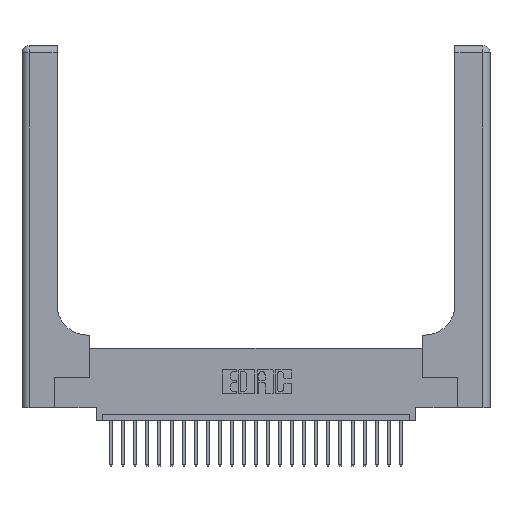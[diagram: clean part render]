
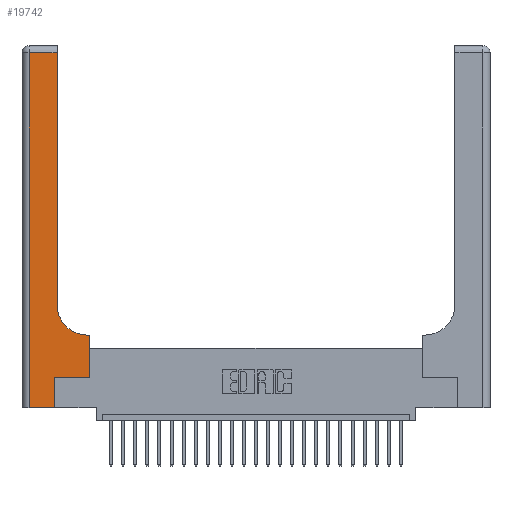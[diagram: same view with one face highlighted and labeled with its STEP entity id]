
A CAD part, top view. The second image highlights one B-rep face of the part: STEP entity #19742.
In plain terms, the highlighted planar face has unit normal (0, 0, 1).
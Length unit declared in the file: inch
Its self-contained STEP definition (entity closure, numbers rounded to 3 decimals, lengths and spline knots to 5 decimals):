
#167 = DIRECTION ( 'NONE',  ( -1., 0., 0. ) ) ;
#295 = AXIS2_PLACEMENT_3D ( 'NONE', #11099, #20944, #6883 ) ;
#512 = DIRECTION ( 'NONE',  ( 0., 1., 0. ) ) ;
#840 = DIRECTION ( 'NONE',  ( 0., 1., 0. ) ) ;
#987 = ORIENTED_EDGE ( 'NONE', *, *, #4149, .T. ) ;
#1193 = EDGE_CURVE ( 'NONE', #26446, #3257, #25566, .T. ) ;
#1522 = CARTESIAN_POINT ( 'NONE',  ( 0.269, 0.25, 0.37 ) ) ;
#2571 = LINE ( 'NONE', #17048, #23633 ) ;
#2656 = LINE ( 'NONE', #3651, #12522 ) ;
#3183 = EDGE_CURVE ( 'NONE', #15405, #6503, #21629, .T. ) ;
#3257 = VERTEX_POINT ( 'NONE', #11018 ) ;
#3651 = CARTESIAN_POINT ( 'NONE',  ( 0., 0., 0.37 ) ) ;
#4149 = EDGE_CURVE ( 'NONE', #6503, #6790, #21908, .T. ) ;
#5219 = ORIENTED_EDGE ( 'NONE', *, *, #18843, .T. ) ;
#5277 = ORIENTED_EDGE ( 'NONE', *, *, #26158, .T. ) ;
#5374 = VECTOR ( 'NONE', #512, 39.37008 ) ;
#5644 = DIRECTION ( 'NONE',  ( 1., 0., 0. ) ) ;
#5876 = EDGE_CURVE ( 'NONE', #23414, #14457, #11928, .T. ) ;
#6503 = VERTEX_POINT ( 'NONE', #17704 ) ;
#6790 = VERTEX_POINT ( 'NONE', #14554 ) ;
#6883 = DIRECTION ( 'NONE',  ( -1., 0., 0. ) ) ;
#7568 = DIRECTION ( 'NONE',  ( 0., -1., 0. ) ) ;
#7780 = EDGE_LOOP ( 'NONE', ( #5277, #13951, #21192, #15056, #25373, #987, #13363, #12437, #5219 ) ) ;
#9045 = CARTESIAN_POINT ( 'NONE',  ( 0.2915, 3., 0.37 ) ) ;
#9907 = VECTOR ( 'NONE', #167, 39.37008 ) ;
#10190 = CARTESIAN_POINT ( 'NONE',  ( 0.2915, 0.6, 0.37 ) ) ;
#11018 = CARTESIAN_POINT ( 'NONE',  ( 0.06, 0., 0.37 ) ) ;
#11099 = CARTESIAN_POINT ( 'NONE',  ( 0., 3., 0.37 ) ) ;
#11488 = LINE ( 'NONE', #9045, #25564 ) ;
#11489 = VECTOR ( 'NONE', #7568, 39.37008 ) ;
#11928 = LINE ( 'NONE', #10190, #20907 ) ;
#12132 = CARTESIAN_POINT ( 'NONE',  ( 0.5585, 0.6, 0.37 ) ) ;
#12437 = ORIENTED_EDGE ( 'NONE', *, *, #5876, .T. ) ;
#12522 = VECTOR ( 'NONE', #13855, 39.37008 ) ;
#12694 = CARTESIAN_POINT ( 'NONE',  ( 0.269, 0., 0.37 ) ) ;
#12975 = PLANE ( 'NONE',  #295 ) ;
#13363 = ORIENTED_EDGE ( 'NONE', *, *, #26314, .T. ) ;
#13855 = DIRECTION ( 'NONE',  ( 1., 0., 0. ) ) ;
#13951 = ORIENTED_EDGE ( 'NONE', *, *, #24109, .T. ) ;
#14452 = CARTESIAN_POINT ( 'NONE',  ( 0.5415, 0.85, 0.37 ) ) ;
#14457 = VERTEX_POINT ( 'NONE', #24742 ) ;
#14554 = CARTESIAN_POINT ( 'NONE',  ( 0.5585, 0.25, 0.37 ) ) ;
#15056 = ORIENTED_EDGE ( 'NONE', *, *, #22880, .T. ) ;
#15338 = LINE ( 'NONE', #26398, #9907 ) ;
#15405 = VERTEX_POINT ( 'NONE', #21794 ) ;
#17048 = CARTESIAN_POINT ( 'NONE',  ( 0.5585, 0.25, 0.37 ) ) ;
#17207 = CIRCLE ( 'NONE', #22969, 0.25 ) ;
#17704 = CARTESIAN_POINT ( 'NONE',  ( 0.269, 0.25, 0.37 ) ) ;
#17805 = FACE_OUTER_BOUND ( 'NONE', #7780, .T. ) ;
#18213 = VERTEX_POINT ( 'NONE', #18227 ) ;
#18227 = CARTESIAN_POINT ( 'NONE',  ( 0.2915, 2.94, 0.37 ) ) ;
#18654 = DIRECTION ( 'NONE',  ( 0., 0., -1. ) ) ;
#18843 = EDGE_CURVE ( 'NONE', #14457, #23407, #17207, .T. ) ;
#19742 = ADVANCED_FACE ( 'NONE', ( #17805 ), #12975, .F. ) ;
#20171 = CARTESIAN_POINT ( 'NONE',  ( 0.06, 2.94, 0.37 ) ) ;
#20478 = DIRECTION ( 'NONE',  ( -1., 0., 0. ) ) ;
#20541 = DIRECTION ( 'NONE',  ( 1., 0., 0. ) ) ;
#20907 = VECTOR ( 'NONE', #20478, 39.37008 ) ;
#20944 = DIRECTION ( 'NONE',  ( 0., 0., -1. ) ) ;
#21192 = ORIENTED_EDGE ( 'NONE', *, *, #1193, .T. ) ;
#21482 = CARTESIAN_POINT ( 'NONE',  ( 0.06, 3., 0.37 ) ) ;
#21629 = LINE ( 'NONE', #12694, #5374 ) ;
#21714 = DIRECTION ( 'NONE',  ( 0., 1., 0. ) ) ;
#21794 = CARTESIAN_POINT ( 'NONE',  ( 0.269, 0., 0.37 ) ) ;
#21908 = LINE ( 'NONE', #1522, #25117 ) ;
#22880 = EDGE_CURVE ( 'NONE', #3257, #15405, #2656, .T. ) ;
#22969 = AXIS2_PLACEMENT_3D ( 'NONE', #14452, #18654, #20541 ) ;
#23407 = VERTEX_POINT ( 'NONE', #24371 ) ;
#23414 = VERTEX_POINT ( 'NONE', #12132 ) ;
#23633 = VECTOR ( 'NONE', #21714, 39.37008 ) ;
#24109 = EDGE_CURVE ( 'NONE', #18213, #26446, #15338, .T. ) ;
#24371 = CARTESIAN_POINT ( 'NONE',  ( 0.2915, 0.85, 0.37 ) ) ;
#24742 = CARTESIAN_POINT ( 'NONE',  ( 0.5415, 0.6, 0.37 ) ) ;
#25117 = VECTOR ( 'NONE', #5644, 39.37008 ) ;
#25373 = ORIENTED_EDGE ( 'NONE', *, *, #3183, .T. ) ;
#25564 = VECTOR ( 'NONE', #840, 39.37008 ) ;
#25566 = LINE ( 'NONE', #21482, #11489 ) ;
#26158 = EDGE_CURVE ( 'NONE', #23407, #18213, #11488, .T. ) ;
#26314 = EDGE_CURVE ( 'NONE', #6790, #23414, #2571, .T. ) ;
#26398 = CARTESIAN_POINT ( 'NONE',  ( 0., 2.94, 0.37 ) ) ;
#26446 = VERTEX_POINT ( 'NONE', #20171 ) ;
